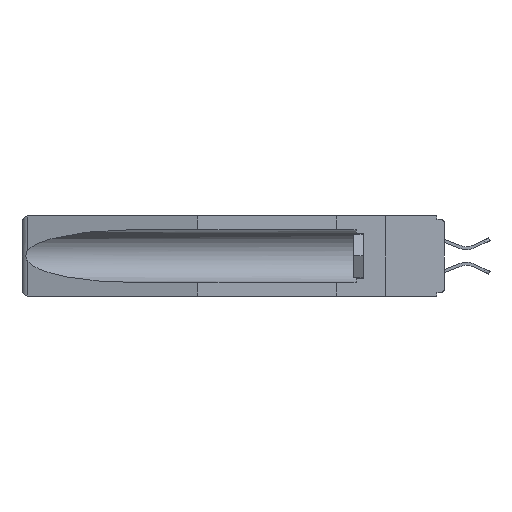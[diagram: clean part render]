
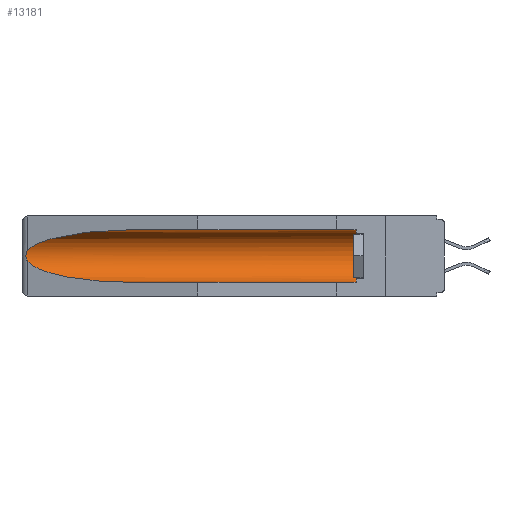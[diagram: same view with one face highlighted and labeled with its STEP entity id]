
A CAD part, left-side view. The second image highlights one B-rep face of the part: STEP entity #13181.
In plain terms, the highlighted cylindrical face has radius 2.857 mm (diameter 5.715 mm), a partial arc.
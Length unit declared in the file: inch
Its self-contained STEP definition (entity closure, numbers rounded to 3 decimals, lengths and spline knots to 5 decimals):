
#1369 = DIRECTION ( 'NONE',  ( 0., 1., 0. ) ) ;
#1453 = EDGE_LOOP ( 'NONE', ( #15495, #13477, #3052, #2790, #11046, #17356 ) ) ;
#2022 = CARTESIAN_POINT ( 'NONE',  ( 0.2675, 1.53308, -0.16763 ) ) ;
#2322 = CARTESIAN_POINT ( 'NONE',  ( 0.2675, 1.53308, -0.17534 ) ) ;
#2329 = CARTESIAN_POINT ( 'NONE',  ( 0.155, 0.126, -0.059 ) ) ;
#2581 = CARTESIAN_POINT ( 'NONE',  ( 0.155, 1.07973, -0.284 ) ) ;
#2677 = CARTESIAN_POINT ( 'NONE',  ( 0.155, 0.126, -0.284 ) ) ;
#2718 = EDGE_CURVE ( 'NONE', #12193, #9631, #18138, .T. ) ;
#2790 = ORIENTED_EDGE ( 'NONE', *, *, #2718, .F. ) ;
#2923 = B_SPLINE_CURVE_WITH_KNOTS ( 'NONE', 3,
 ( #5360, #17158, #14188, #19753, #2022, #2322, #6468, #7319, #6564, #6436 ),
 .UNSPECIFIED., .F., .F.,
 ( 4, 2, 2, 2, 4 ),
 ( 0., 0.00029, 0.00058, 0.00087, 0.00117 ),
 .UNSPECIFIED. ) ;
#3052 = ORIENTED_EDGE ( 'NONE', *, *, #3703, .T. ) ;
#3103 = CARTESIAN_POINT ( 'NONE',  ( 0.26537, 1.52718, -0.19328 ) ) ;
#3473 = AXIS2_PLACEMENT_3D ( 'NONE', #15594, #12608, #15737 ) ;
#3492 = CARTESIAN_POINT ( 'NONE',  ( 0.21114, 1.30732, -0.059 ) ) ;
#3619 = EDGE_CURVE ( 'NONE', #11637, #4036, #14163, .T. ) ;
#3662 = VECTOR ( 'NONE', #1369, 39.37008 ) ;
#3703 = EDGE_CURVE ( 'NONE', #16087, #9631, #4420, .T. ) ;
#4036 = VERTEX_POINT ( 'NONE', #9336 ) ;
#4420 =( BOUNDED_CURVE ( )  B_SPLINE_CURVE ( 3, ( #13163, #6845, #10405, #2581 ),
 .UNSPECIFIED., .F., .F. ) 
 B_SPLINE_CURVE_WITH_KNOTS ( ( 4, 4 ),
 ( 0.1948, 1.5708 ),
 .UNSPECIFIED. ) 
 CURVE ( )  GEOMETRIC_REPRESENTATION_ITEM ( )  RATIONAL_B_SPLINE_CURVE ( ( 1., 0.848, 0.848, 1. ) ) 
 REPRESENTATION_ITEM ( '' )  );
#5360 = CARTESIAN_POINT ( 'NONE',  ( 0.26537, 1.52718, -0.14972 ) ) ;
#6231 = AXIS2_PLACEMENT_3D ( 'NONE', #13515, #12173, #9121 ) ;
#6436 = CARTESIAN_POINT ( 'NONE',  ( 0.26537, 1.52718, -0.19328 ) ) ;
#6468 = CARTESIAN_POINT ( 'NONE',  ( 0.2673, 1.53269, -0.17917 ) ) ;
#6564 = CARTESIAN_POINT ( 'NONE',  ( 0.26597, 1.5296, -0.19026 ) ) ;
#6612 = CARTESIAN_POINT ( 'NONE',  ( 0.25451, 1.48313, -0.09465 ) ) ;
#6810 = CARTESIAN_POINT ( 'NONE',  ( 0.155, 1.07973, -0.059 ) ) ;
#6845 = CARTESIAN_POINT ( 'NONE',  ( 0.25451, 1.48313, -0.24835 ) ) ;
#6862 = EDGE_CURVE ( 'NONE', #12193, #11637, #8943, .T. ) ;
#7319 = CARTESIAN_POINT ( 'NONE',  ( 0.26655, 1.53094, -0.18657 ) ) ;
#8078 = DIRECTION ( 'NONE',  ( 0., 1., 0. ) ) ;
#8148 = CYLINDRICAL_SURFACE ( 'NONE', #6231, 0.1125 ) ;
#8437 = CARTESIAN_POINT ( 'NONE',  ( 0.26537, 1.52718, -0.14972 ) ) ;
#8943 = CIRCLE ( 'NONE', #3473, 0.1125 ) ;
#9121 = DIRECTION ( 'NONE',  ( 0., 0., 1. ) ) ;
#9336 = CARTESIAN_POINT ( 'NONE',  ( 0.155, 1.07973, -0.059 ) ) ;
#9479 = CARTESIAN_POINT ( 'NONE',  ( 0.155, -0.30754, -0.284 ) ) ;
#9631 = VERTEX_POINT ( 'NONE', #10199 ) ;
#10199 = CARTESIAN_POINT ( 'NONE',  ( 0.155, 1.07973, -0.284 ) ) ;
#10405 = CARTESIAN_POINT ( 'NONE',  ( 0.21114, 1.30732, -0.284 ) ) ;
#10628 = FACE_OUTER_BOUND ( 'NONE', #1453, .T. ) ;
#11046 = ORIENTED_EDGE ( 'NONE', *, *, #6862, .T. ) ;
#11637 = VERTEX_POINT ( 'NONE', #2329 ) ;
#11983 = CARTESIAN_POINT ( 'NONE',  ( 0.26537, 1.52718, -0.14972 ) ) ;
#12173 = DIRECTION ( 'NONE',  ( 0., 1., 0. ) ) ;
#12193 = VERTEX_POINT ( 'NONE', #2677 ) ;
#12608 = DIRECTION ( 'NONE',  ( 0., -1., 0. ) ) ;
#13163 = CARTESIAN_POINT ( 'NONE',  ( 0.26537, 1.52718, -0.19328 ) ) ;
#13181 = ADVANCED_FACE ( 'NONE', ( #10628 ), #8148, .F. ) ;
#13477 = ORIENTED_EDGE ( 'NONE', *, *, #13956, .T. ) ;
#13515 = CARTESIAN_POINT ( 'NONE',  ( 0.155, -0.30754, -0.1715 ) ) ;
#13956 = EDGE_CURVE ( 'NONE', #19882, #16087, #2923, .T. ) ;
#14163 = LINE ( 'NONE', #18688, #3662 ) ;
#14188 = CARTESIAN_POINT ( 'NONE',  ( 0.26654, 1.53092, -0.15636 ) ) ;
#15495 = ORIENTED_EDGE ( 'NONE', *, *, #16834, .T. ) ;
#15594 = CARTESIAN_POINT ( 'NONE',  ( 0.155, 0.126, -0.1715 ) ) ;
#15737 = DIRECTION ( 'NONE',  ( 0., 0., 1. ) ) ;
#16087 = VERTEX_POINT ( 'NONE', #3103 ) ;
#16834 = EDGE_CURVE ( 'NONE', #4036, #19882, #19611, .T. ) ;
#17158 = CARTESIAN_POINT ( 'NONE',  ( 0.26597, 1.52961, -0.15275 ) ) ;
#17356 = ORIENTED_EDGE ( 'NONE', *, *, #3619, .T. ) ;
#17424 = VECTOR ( 'NONE', #8078, 39.37008 ) ;
#18138 = LINE ( 'NONE', #9479, #17424 ) ;
#18688 = CARTESIAN_POINT ( 'NONE',  ( 0.155, -0.30754, -0.059 ) ) ;
#19611 =( BOUNDED_CURVE ( )  B_SPLINE_CURVE ( 3, ( #6810, #3492, #6612, #8437 ),
 .UNSPECIFIED., .F., .F. ) 
 B_SPLINE_CURVE_WITH_KNOTS ( ( 4, 4 ),
 ( 4.71239, 6.08839 ),
 .UNSPECIFIED. ) 
 CURVE ( )  GEOMETRIC_REPRESENTATION_ITEM ( )  RATIONAL_B_SPLINE_CURVE ( ( 1., 0.848, 0.848, 1. ) ) 
 REPRESENTATION_ITEM ( '' )  );
#19753 = CARTESIAN_POINT ( 'NONE',  ( 0.2673, 1.5327, -0.16383 ) ) ;
#19882 = VERTEX_POINT ( 'NONE', #11983 ) ;
